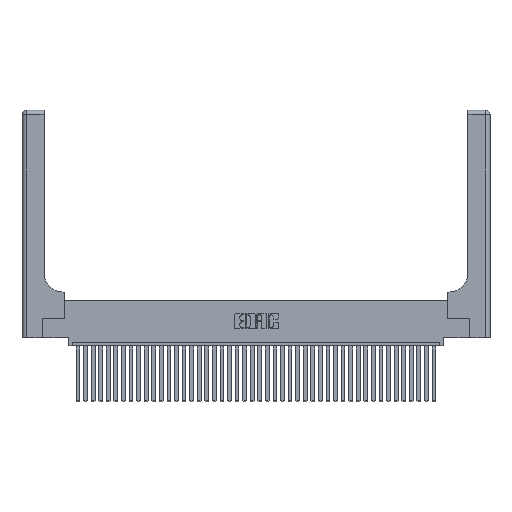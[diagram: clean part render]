
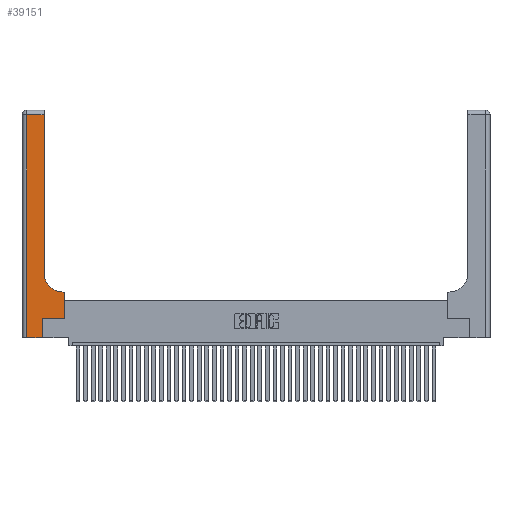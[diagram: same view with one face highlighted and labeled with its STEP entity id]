
A CAD part, top view. The second image highlights one B-rep face of the part: STEP entity #39151.
In plain terms, the highlighted planar face has unit normal (0, 0, 1).
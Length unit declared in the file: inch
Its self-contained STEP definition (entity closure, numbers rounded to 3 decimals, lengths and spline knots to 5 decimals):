
#934 = EDGE_CURVE ( 'NONE', #9009, #9655, #15465, .T. ) ;
#1206 = CARTESIAN_POINT ( 'NONE',  ( 0.5585, 0.25, 0.37 ) ) ;
#3115 = DIRECTION ( 'NONE',  ( 1., 0., 0. ) ) ;
#3150 = EDGE_CURVE ( 'NONE', #9655, #39415, #26446, .T. ) ;
#3168 = PLANE ( 'NONE',  #38754 ) ;
#3198 = EDGE_CURVE ( 'NONE', #13006, #4477, #21601, .T. ) ;
#3690 = ORIENTED_EDGE ( 'NONE', *, *, #9088, .T. ) ;
#3732 = VERTEX_POINT ( 'NONE', #34773 ) ;
#4170 = DIRECTION ( 'NONE',  ( 0., -1., 0. ) ) ;
#4327 = AXIS2_PLACEMENT_3D ( 'NONE', #30158, #17761, #33136 ) ;
#4477 = VERTEX_POINT ( 'NONE', #7608 ) ;
#4841 = EDGE_CURVE ( 'NONE', #39415, #3732, #22854, .T. ) ;
#5289 = VERTEX_POINT ( 'NONE', #25096 ) ;
#5528 = EDGE_LOOP ( 'NONE', ( #6923, #27484, #27806, #6287, #35928, #7537, #38620, #28810, #3690 ) ) ;
#5683 = CIRCLE ( 'NONE', #4327, 0.25 ) ;
#5798 = CARTESIAN_POINT ( 'NONE',  ( 0.2915, 0.6, 0.37 ) ) ;
#6287 = ORIENTED_EDGE ( 'NONE', *, *, #28113, .T. ) ;
#6730 = CARTESIAN_POINT ( 'NONE',  ( 0., 2.94, 0.37 ) ) ;
#6875 = CARTESIAN_POINT ( 'NONE',  ( 0.269, 0., 0.37 ) ) ;
#6923 = ORIENTED_EDGE ( 'NONE', *, *, #3198, .T. ) ;
#7010 = LINE ( 'NONE', #6730, #11972 ) ;
#7022 = CARTESIAN_POINT ( 'NONE',  ( 0.06, 3., 0.37 ) ) ;
#7116 = VECTOR ( 'NONE', #12767, 39.37008 ) ;
#7537 = ORIENTED_EDGE ( 'NONE', *, *, #3150, .T. ) ;
#7608 = CARTESIAN_POINT ( 'NONE',  ( 0.2915, 2.94, 0.37 ) ) ;
#8086 = CARTESIAN_POINT ( 'NONE',  ( 0.2915, 0.85, 0.37 ) ) ;
#8140 = LINE ( 'NONE', #7022, #19348 ) ;
#9009 = VERTEX_POINT ( 'NONE', #19818 ) ;
#9067 = VECTOR ( 'NONE', #3115, 39.37008 ) ;
#9088 = EDGE_CURVE ( 'NONE', #35610, #13006, #5683, .T. ) ;
#9655 = VERTEX_POINT ( 'NONE', #24453 ) ;
#11575 = DIRECTION ( 'NONE',  ( 0., 1., 0. ) ) ;
#11972 = VECTOR ( 'NONE', #31280, 39.37008 ) ;
#12096 = DIRECTION ( 'NONE',  ( -1., 0., 0. ) ) ;
#12742 = CARTESIAN_POINT ( 'NONE',  ( 0.2915, 3., 0.37 ) ) ;
#12767 = DIRECTION ( 'NONE',  ( 0., 1., 0. ) ) ;
#13006 = VERTEX_POINT ( 'NONE', #8086 ) ;
#14948 = VECTOR ( 'NONE', #12096, 39.37008 ) ;
#15465 = LINE ( 'NONE', #6875, #7116 ) ;
#16338 = LINE ( 'NONE', #18089, #9067 ) ;
#17761 = DIRECTION ( 'NONE',  ( 0., 0., -1. ) ) ;
#18089 = CARTESIAN_POINT ( 'NONE',  ( 0., 0., 0.37 ) ) ;
#18653 = DIRECTION ( 'NONE',  ( 1., 0., 0. ) ) ;
#19348 = VECTOR ( 'NONE', #4170, 39.37008 ) ;
#19818 = CARTESIAN_POINT ( 'NONE',  ( 0.269, 0., 0.37 ) ) ;
#20628 = VECTOR ( 'NONE', #18653, 39.37008 ) ;
#21601 = LINE ( 'NONE', #12742, #28400 ) ;
#21763 = LINE ( 'NONE', #5798, #14948 ) ;
#21787 = EDGE_CURVE ( 'NONE', #5289, #31947, #8140, .T. ) ;
#21983 = DIRECTION ( 'NONE',  ( 0., 0., -1. ) ) ;
#22107 = CARTESIAN_POINT ( 'NONE',  ( 0., 3., 0.37 ) ) ;
#22854 = LINE ( 'NONE', #36949, #39516 ) ;
#23477 = FACE_OUTER_BOUND ( 'NONE', #5528, .T. ) ;
#24453 = CARTESIAN_POINT ( 'NONE',  ( 0.269, 0.25, 0.37 ) ) ;
#24899 = CARTESIAN_POINT ( 'NONE',  ( 0.269, 0.25, 0.37 ) ) ;
#25096 = CARTESIAN_POINT ( 'NONE',  ( 0.06, 2.94, 0.37 ) ) ;
#26444 = CARTESIAN_POINT ( 'NONE',  ( 0.5415, 0.6, 0.37 ) ) ;
#26446 = LINE ( 'NONE', #24899, #20628 ) ;
#27484 = ORIENTED_EDGE ( 'NONE', *, *, #28499, .T. ) ;
#27675 = EDGE_CURVE ( 'NONE', #3732, #35610, #21763, .T. ) ;
#27806 = ORIENTED_EDGE ( 'NONE', *, *, #21787, .T. ) ;
#28113 = EDGE_CURVE ( 'NONE', #31947, #9009, #16338, .T. ) ;
#28400 = VECTOR ( 'NONE', #34188, 39.37008 ) ;
#28499 = EDGE_CURVE ( 'NONE', #4477, #5289, #7010, .T. ) ;
#28810 = ORIENTED_EDGE ( 'NONE', *, *, #27675, .T. ) ;
#30158 = CARTESIAN_POINT ( 'NONE',  ( 0.5415, 0.85, 0.37 ) ) ;
#31280 = DIRECTION ( 'NONE',  ( -1., 0., 0. ) ) ;
#31472 = DIRECTION ( 'NONE',  ( -1., 0., 0. ) ) ;
#31947 = VERTEX_POINT ( 'NONE', #35627 ) ;
#33136 = DIRECTION ( 'NONE',  ( 1., 0., 0. ) ) ;
#34188 = DIRECTION ( 'NONE',  ( 0., 1., 0. ) ) ;
#34773 = CARTESIAN_POINT ( 'NONE',  ( 0.5585, 0.6, 0.37 ) ) ;
#35610 = VERTEX_POINT ( 'NONE', #26444 ) ;
#35627 = CARTESIAN_POINT ( 'NONE',  ( 0.06, 0., 0.37 ) ) ;
#35928 = ORIENTED_EDGE ( 'NONE', *, *, #934, .T. ) ;
#36949 = CARTESIAN_POINT ( 'NONE',  ( 0.5585, 0.25, 0.37 ) ) ;
#38620 = ORIENTED_EDGE ( 'NONE', *, *, #4841, .T. ) ;
#38754 = AXIS2_PLACEMENT_3D ( 'NONE', #22107, #21983, #31472 ) ;
#39151 = ADVANCED_FACE ( 'NONE', ( #23477 ), #3168, .F. ) ;
#39415 = VERTEX_POINT ( 'NONE', #1206 ) ;
#39516 = VECTOR ( 'NONE', #11575, 39.37008 ) ;
